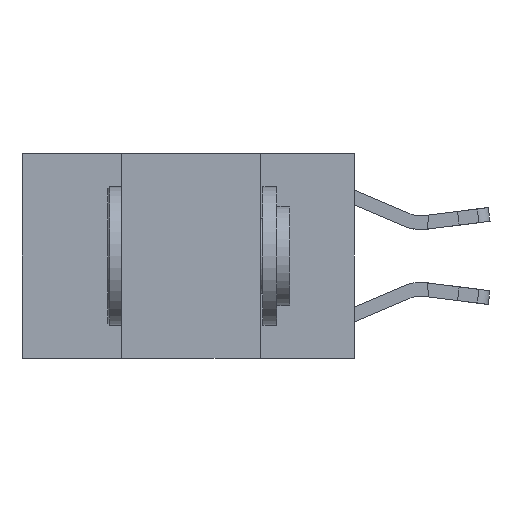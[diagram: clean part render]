
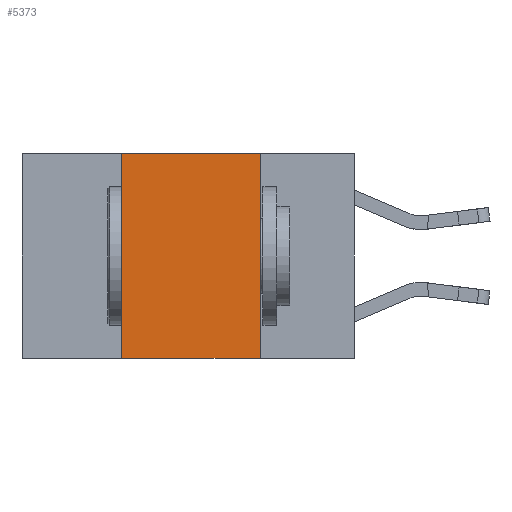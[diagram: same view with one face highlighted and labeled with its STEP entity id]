
A CAD part, left-side view. The second image highlights one B-rep face of the part: STEP entity #5373.
In plain terms, the highlighted planar face has unit normal (-1, 0, 0).
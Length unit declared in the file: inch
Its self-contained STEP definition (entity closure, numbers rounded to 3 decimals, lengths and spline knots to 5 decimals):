
#1806 = EDGE_CURVE ( 'NONE', #6534, #3075, #17189, .T. ) ;
#2993 = CARTESIAN_POINT ( 'NONE',  ( 0., 0.42, 0. ) ) ;
#3075 = VERTEX_POINT ( 'NONE', #18944 ) ;
#3460 = DIRECTION ( 'NONE',  ( 0., 0., -1. ) ) ;
#3892 = VECTOR ( 'NONE', #12663, 39.37008 ) ;
#4028 = DIRECTION ( 'NONE',  ( 0., -1., 0. ) ) ;
#4166 = ORIENTED_EDGE ( 'NONE', *, *, #19253, .F. ) ;
#5373 = ADVANCED_FACE ( 'NONE', ( #10154 ), #13962, .F. ) ;
#6534 = VERTEX_POINT ( 'NONE', #8274 ) ;
#6639 = DIRECTION ( 'NONE',  ( 0., 0., -1. ) ) ;
#6940 = CARTESIAN_POINT ( 'NONE',  ( 0., 0.6, 0. ) ) ;
#6980 = VERTEX_POINT ( 'NONE', #19964 ) ;
#8274 = CARTESIAN_POINT ( 'NONE',  ( 0., 0.17, 0. ) ) ;
#8599 = LINE ( 'NONE', #19596, #3892 ) ;
#8705 = VERTEX_POINT ( 'NONE', #20866 ) ;
#10029 = DIRECTION ( 'NONE',  ( 0., 0., 1. ) ) ;
#10154 = FACE_OUTER_BOUND ( 'NONE', #21702, .T. ) ;
#10550 = EDGE_CURVE ( 'NONE', #6980, #3075, #8599, .T. ) ;
#12663 = DIRECTION ( 'NONE',  ( 0., -1., 0. ) ) ;
#12894 = CARTESIAN_POINT ( 'NONE',  ( 0., 0.6, 0. ) ) ;
#13558 = ORIENTED_EDGE ( 'NONE', *, *, #10550, .T. ) ;
#13962 = PLANE ( 'NONE',  #22392 ) ;
#14043 = DIRECTION ( 'NONE',  ( 1., 0., 0. ) ) ;
#15428 = CARTESIAN_POINT ( 'NONE',  ( 0., 0.17, 0. ) ) ;
#17189 = LINE ( 'NONE', #15428, #20756 ) ;
#17830 = VECTOR ( 'NONE', #4028, 39.37008 ) ;
#18393 = EDGE_CURVE ( 'NONE', #8705, #6534, #21917, .T. ) ;
#18944 = CARTESIAN_POINT ( 'NONE',  ( 0., 0.17, -0.37 ) ) ;
#19253 = EDGE_CURVE ( 'NONE', #6980, #8705, #21973, .T. ) ;
#19596 = CARTESIAN_POINT ( 'NONE',  ( 0., 0.6, -0.37 ) ) ;
#19964 = CARTESIAN_POINT ( 'NONE',  ( 0., 0.42, -0.37 ) ) ;
#20756 = VECTOR ( 'NONE', #6639, 39.37008 ) ;
#20866 = CARTESIAN_POINT ( 'NONE',  ( 0., 0.42, 0. ) ) ;
#21424 = VECTOR ( 'NONE', #10029, 39.37008 ) ;
#21702 = EDGE_LOOP ( 'NONE', ( #21810, #22353, #4166, #13558 ) ) ;
#21810 = ORIENTED_EDGE ( 'NONE', *, *, #1806, .F. ) ;
#21917 = LINE ( 'NONE', #12894, #17830 ) ;
#21973 = LINE ( 'NONE', #2993, #21424 ) ;
#22353 = ORIENTED_EDGE ( 'NONE', *, *, #18393, .F. ) ;
#22392 = AXIS2_PLACEMENT_3D ( 'NONE', #6940, #14043, #3460 ) ;
